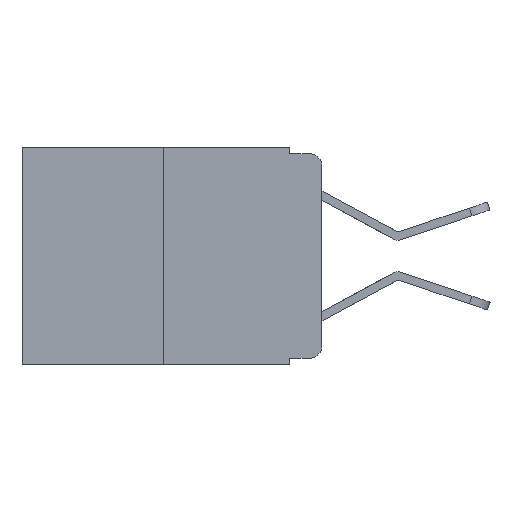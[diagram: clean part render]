
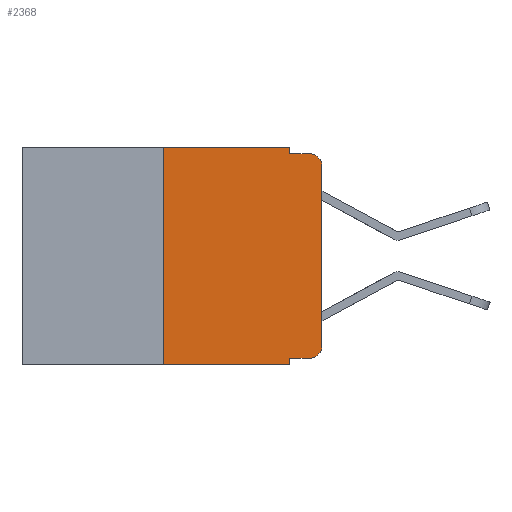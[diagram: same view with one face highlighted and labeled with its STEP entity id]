
A CAD part, left-side view. The second image highlights one B-rep face of the part: STEP entity #2368.
In plain terms, the highlighted planar face has unit normal (-1, 0, 0).
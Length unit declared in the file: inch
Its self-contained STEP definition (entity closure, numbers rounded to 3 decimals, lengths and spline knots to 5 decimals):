
#18 = VERTEX_POINT ( 'NONE', #13277 ) ;
#536 = DIRECTION ( 'NONE',  ( 0., -1., 0. ) ) ;
#691 = DIRECTION ( 'NONE',  ( -1., 0., 0. ) ) ;
#804 = CARTESIAN_POINT ( 'NONE',  ( 0., 0.02, -0.313 ) ) ;
#958 = VECTOR ( 'NONE', #12471, 39.37008 ) ;
#1097 = DIRECTION ( 'NONE',  ( 0., -1., 0. ) ) ;
#1112 = LINE ( 'NONE', #5559, #12010 ) ;
#1511 = AXIS2_PLACEMENT_3D ( 'NONE', #11177, #2156, #14547 ) ;
#1584 = AXIS2_PLACEMENT_3D ( 'NONE', #804, #691, #8597 ) ;
#1624 = CARTESIAN_POINT ( 'NONE',  ( 0., 0.473, -0.343 ) ) ;
#1712 = ORIENTED_EDGE ( 'NONE', *, *, #9907, .T. ) ;
#2017 = CARTESIAN_POINT ( 'NONE',  ( 0., 0., -0.313 ) ) ;
#2156 = DIRECTION ( 'NONE',  ( 1., 0., 0. ) ) ;
#2336 = CARTESIAN_POINT ( 'NONE',  ( 0., 0.051, -0.333 ) ) ;
#2368 = ADVANCED_FACE ( 'NONE', ( #3088 ), #13321, .F. ) ;
#3088 = FACE_OUTER_BOUND ( 'NONE', #13840, .T. ) ;
#3205 = ORIENTED_EDGE ( 'NONE', *, *, #12782, .F. ) ;
#3742 = LINE ( 'NONE', #14538, #12549 ) ;
#3825 = EDGE_CURVE ( 'NONE', #4085, #14417, #1112, .T. ) ;
#3905 = CARTESIAN_POINT ( 'NONE',  ( 0., 0.051, -0.01 ) ) ;
#3914 = VERTEX_POINT ( 'NONE', #10463 ) ;
#3972 = LINE ( 'NONE', #5439, #5882 ) ;
#4085 = VERTEX_POINT ( 'NONE', #3905 ) ;
#4332 = LINE ( 'NONE', #13541, #10830 ) ;
#4378 = CARTESIAN_POINT ( 'NONE',  ( 0., 0.25, -0.343 ) ) ;
#4388 = VERTEX_POINT ( 'NONE', #7591 ) ;
#4964 = DIRECTION ( 'NONE',  ( -1., 0., 0. ) ) ;
#5108 = LINE ( 'NONE', #5998, #13416 ) ;
#5257 = VECTOR ( 'NONE', #536, 39.37008 ) ;
#5285 = VERTEX_POINT ( 'NONE', #7733 ) ;
#5384 = EDGE_CURVE ( 'NONE', #14392, #6663, #3742, .T. ) ;
#5415 = VECTOR ( 'NONE', #8464, 39.37008 ) ;
#5439 = CARTESIAN_POINT ( 'NONE',  ( 0., 0.473, 0. ) ) ;
#5559 = CARTESIAN_POINT ( 'NONE',  ( 0., 0.051, -0.01 ) ) ;
#5882 = VECTOR ( 'NONE', #8883, 39.37008 ) ;
#5998 = CARTESIAN_POINT ( 'NONE',  ( 0., 0.051, 0. ) ) ;
#6096 = EDGE_CURVE ( 'NONE', #18, #10725, #5108, .T. ) ;
#6663 = VERTEX_POINT ( 'NONE', #9012 ) ;
#6998 = ORIENTED_EDGE ( 'NONE', *, *, #5384, .T. ) ;
#7107 = ORIENTED_EDGE ( 'NONE', *, *, #8188, .T. ) ;
#7426 = VERTEX_POINT ( 'NONE', #4378 ) ;
#7591 = CARTESIAN_POINT ( 'NONE',  ( 0., 0.051, 0. ) ) ;
#7733 = CARTESIAN_POINT ( 'NONE',  ( 0., 0.25, 0. ) ) ;
#7815 = LINE ( 'NONE', #2336, #958 ) ;
#8036 = CIRCLE ( 'NONE', #1584, 0.02 ) ;
#8188 = EDGE_CURVE ( 'NONE', #7426, #10725, #14443, .T. ) ;
#8405 = LINE ( 'NONE', #8565, #5415 ) ;
#8464 = DIRECTION ( 'NONE',  ( 0., 0., -1. ) ) ;
#8565 = CARTESIAN_POINT ( 'NONE',  ( 0., 0.051, 0. ) ) ;
#8597 = DIRECTION ( 'NONE',  ( 0., 0., -1. ) ) ;
#8839 = EDGE_CURVE ( 'NONE', #4388, #4085, #8405, .T. ) ;
#8883 = DIRECTION ( 'NONE',  ( 0., -1., 0. ) ) ;
#9012 = CARTESIAN_POINT ( 'NONE',  ( 0., 0., -0.03 ) ) ;
#9039 = DIRECTION ( 'NONE',  ( 0., 0., 1. ) ) ;
#9418 = EDGE_CURVE ( 'NONE', #3914, #14392, #8036, .T. ) ;
#9704 = ORIENTED_EDGE ( 'NONE', *, *, #6096, .F. ) ;
#9792 = CIRCLE ( 'NONE', #11085, 0.02 ) ;
#9907 = EDGE_CURVE ( 'NONE', #6663, #14417, #9792, .T. ) ;
#10463 = CARTESIAN_POINT ( 'NONE',  ( 0., 0.02, -0.333 ) ) ;
#10725 = VERTEX_POINT ( 'NONE', #11107 ) ;
#10790 = ORIENTED_EDGE ( 'NONE', *, *, #12605, .F. ) ;
#10830 = VECTOR ( 'NONE', #9039, 39.37008 ) ;
#11035 = CARTESIAN_POINT ( 'NONE',  ( 0., 0.02, -0.01 ) ) ;
#11085 = AXIS2_PLACEMENT_3D ( 'NONE', #11716, #4964, #11667 ) ;
#11107 = CARTESIAN_POINT ( 'NONE',  ( 0., 0.051, -0.343 ) ) ;
#11177 = CARTESIAN_POINT ( 'NONE',  ( 0., 0.473, 0. ) ) ;
#11667 = DIRECTION ( 'NONE',  ( 0., 0., -1. ) ) ;
#11716 = CARTESIAN_POINT ( 'NONE',  ( 0., 0.02, -0.03 ) ) ;
#12010 = VECTOR ( 'NONE', #1097, 39.37008 ) ;
#12302 = ORIENTED_EDGE ( 'NONE', *, *, #13986, .T. ) ;
#12471 = DIRECTION ( 'NONE',  ( 0., -1., 0. ) ) ;
#12501 = DIRECTION ( 'NONE',  ( 0., 0., 1. ) ) ;
#12549 = VECTOR ( 'NONE', #12501, 39.37008 ) ;
#12605 = EDGE_CURVE ( 'NONE', #7426, #5285, #4332, .T. ) ;
#12687 = ORIENTED_EDGE ( 'NONE', *, *, #3825, .F. ) ;
#12782 = EDGE_CURVE ( 'NONE', #5285, #4388, #3972, .T. ) ;
#13277 = CARTESIAN_POINT ( 'NONE',  ( 0., 0.051, -0.333 ) ) ;
#13321 = PLANE ( 'NONE',  #1511 ) ;
#13416 = VECTOR ( 'NONE', #13899, 39.37008 ) ;
#13541 = CARTESIAN_POINT ( 'NONE',  ( 0., 0.25, 0. ) ) ;
#13840 = EDGE_LOOP ( 'NONE', ( #6998, #1712, #12687, #14038, #3205, #10790, #7107, #9704, #12302, #14151 ) ) ;
#13899 = DIRECTION ( 'NONE',  ( 0., 0., -1. ) ) ;
#13986 = EDGE_CURVE ( 'NONE', #18, #3914, #7815, .T. ) ;
#14038 = ORIENTED_EDGE ( 'NONE', *, *, #8839, .F. ) ;
#14151 = ORIENTED_EDGE ( 'NONE', *, *, #9418, .T. ) ;
#14392 = VERTEX_POINT ( 'NONE', #2017 ) ;
#14417 = VERTEX_POINT ( 'NONE', #11035 ) ;
#14443 = LINE ( 'NONE', #1624, #5257 ) ;
#14538 = CARTESIAN_POINT ( 'NONE',  ( 0., 0., 0. ) ) ;
#14547 = DIRECTION ( 'NONE',  ( 0., 0., -1. ) ) ;
